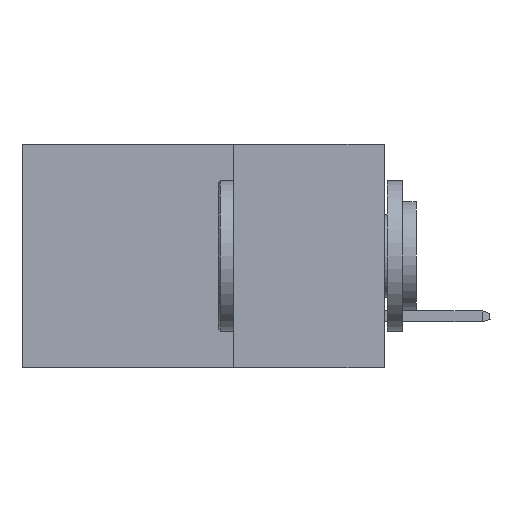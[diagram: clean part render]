
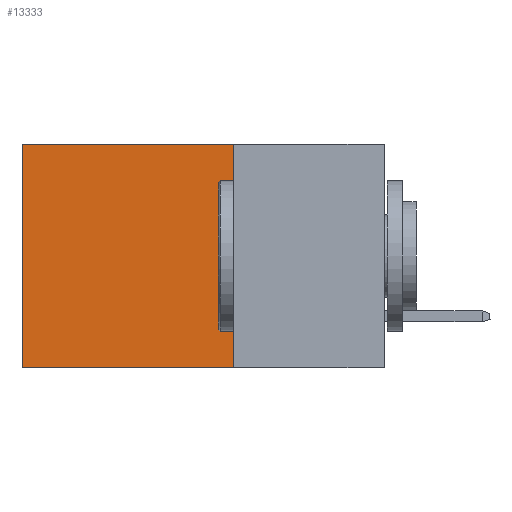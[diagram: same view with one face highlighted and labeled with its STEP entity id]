
A CAD part, left-side view. The second image highlights one B-rep face of the part: STEP entity #13333.
In plain terms, the highlighted planar face has unit normal (-1, 0, 0).
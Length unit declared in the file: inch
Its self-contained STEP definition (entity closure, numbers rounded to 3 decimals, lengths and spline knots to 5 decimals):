
#196 = DIRECTION ( 'NONE',  ( 0., 0., -1. ) ) ;
#238 = ORIENTED_EDGE ( 'NONE', *, *, #8077, .T. ) ;
#866 = AXIS2_PLACEMENT_3D ( 'NONE', #7391, #11499, #196 ) ;
#1729 = EDGE_CURVE ( 'NONE', #9611, #4552, #5623, .T. ) ;
#2045 = ORIENTED_EDGE ( 'NONE', *, *, #7147, .F. ) ;
#2268 = ORIENTED_EDGE ( 'NONE', *, *, #7035, .F. ) ;
#2799 = VERTEX_POINT ( 'NONE', #9091 ) ;
#3070 = CARTESIAN_POINT ( 'NONE',  ( 0.298, 0.25, -0.37 ) ) ;
#3354 = PLANE ( 'NONE',  #866 ) ;
#3724 = CARTESIAN_POINT ( 'NONE',  ( 0.298, 0.25, 0. ) ) ;
#3776 = CARTESIAN_POINT ( 'NONE',  ( 0.298, 0.6, 0. ) ) ;
#4079 = CARTESIAN_POINT ( 'NONE',  ( 0.298, 0.25, 0. ) ) ;
#4482 = CARTESIAN_POINT ( 'NONE',  ( 0.298, 0.6, 0. ) ) ;
#4552 = VERTEX_POINT ( 'NONE', #7225 ) ;
#5623 = LINE ( 'NONE', #3776, #7755 ) ;
#6068 = LINE ( 'NONE', #3070, #11954 ) ;
#7035 = EDGE_CURVE ( 'NONE', #2799, #11078, #12600, .T. ) ;
#7055 = VECTOR ( 'NONE', #13114, 39.37008 ) ;
#7147 = EDGE_CURVE ( 'NONE', #11078, #4552, #6068, .T. ) ;
#7225 = CARTESIAN_POINT ( 'NONE',  ( 0.298, 0.6, -0.37 ) ) ;
#7391 = CARTESIAN_POINT ( 'NONE',  ( 0.298, 0.25, 0. ) ) ;
#7398 = CARTESIAN_POINT ( 'NONE',  ( 0.298, 0.25, -0.37 ) ) ;
#7755 = VECTOR ( 'NONE', #12117, 39.37008 ) ;
#8077 = EDGE_CURVE ( 'NONE', #2799, #9611, #9948, .T. ) ;
#8557 = EDGE_LOOP ( 'NONE', ( #13365, #2045, #2268, #238 ) ) ;
#9091 = CARTESIAN_POINT ( 'NONE',  ( 0.298, 0.25, 0. ) ) ;
#9611 = VERTEX_POINT ( 'NONE', #4482 ) ;
#9948 = LINE ( 'NONE', #4079, #10114 ) ;
#10114 = VECTOR ( 'NONE', #10180, 39.37008 ) ;
#10180 = DIRECTION ( 'NONE',  ( 0., 1., 0. ) ) ;
#10371 = DIRECTION ( 'NONE',  ( 0., 1., 0. ) ) ;
#11078 = VERTEX_POINT ( 'NONE', #7398 ) ;
#11499 = DIRECTION ( 'NONE',  ( 1., 0., 0. ) ) ;
#11954 = VECTOR ( 'NONE', #10371, 39.37008 ) ;
#12117 = DIRECTION ( 'NONE',  ( 0., 0., -1. ) ) ;
#12600 = LINE ( 'NONE', #3724, #7055 ) ;
#13114 = DIRECTION ( 'NONE',  ( 0., 0., -1. ) ) ;
#13276 = FACE_OUTER_BOUND ( 'NONE', #8557, .T. ) ;
#13333 = ADVANCED_FACE ( 'NONE', ( #13276 ), #3354, .F. ) ;
#13365 = ORIENTED_EDGE ( 'NONE', *, *, #1729, .T. ) ;
